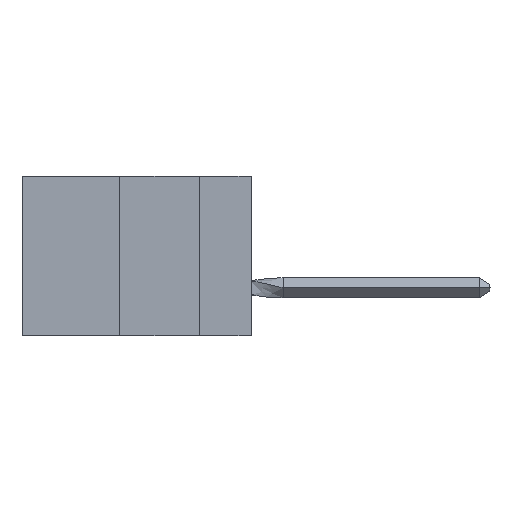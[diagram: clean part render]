
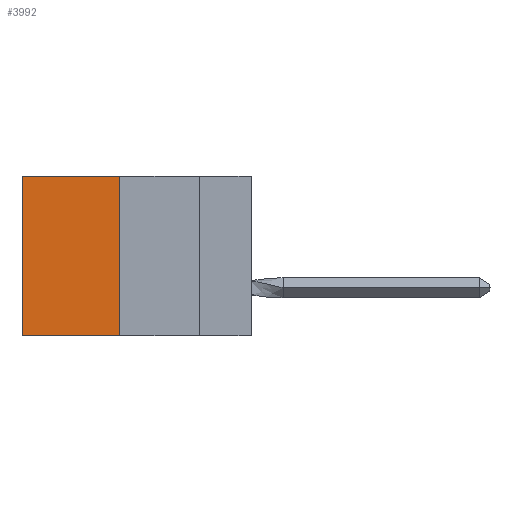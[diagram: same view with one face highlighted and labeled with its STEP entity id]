
A CAD part, left-side view. The second image highlights one B-rep face of the part: STEP entity #3992.
In plain terms, the highlighted planar face has unit normal (-1, 0, 0).
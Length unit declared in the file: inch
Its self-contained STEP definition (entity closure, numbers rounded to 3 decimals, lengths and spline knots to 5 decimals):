
#480 = VERTEX_POINT ( 'NONE', #12824 ) ;
#932 = PLANE ( 'NONE',  #18808 ) ;
#1014 = VERTEX_POINT ( 'NONE', #12391 ) ;
#2527 = ORIENTED_EDGE ( 'NONE', *, *, #12976, .T. ) ;
#2913 = DIRECTION ( 'NONE',  ( 0., 1., 0. ) ) ;
#2968 = CARTESIAN_POINT ( 'NONE',  ( 0.305, 0.413, -0.5 ) ) ;
#3451 = LINE ( 'NONE', #14095, #17153 ) ;
#3831 = DIRECTION ( 'NONE',  ( 0., 0., -1. ) ) ;
#3992 = ADVANCED_FACE ( 'NONE', ( #8481 ), #932, .F. ) ;
#5129 = CARTESIAN_POINT ( 'NONE',  ( 0.305, 0.413, -0.5 ) ) ;
#5790 = LINE ( 'NONE', #5129, #18299 ) ;
#6996 = ORIENTED_EDGE ( 'NONE', *, *, #18344, .F. ) ;
#7766 = DIRECTION ( 'NONE',  ( 0., 1., 0. ) ) ;
#8481 = FACE_OUTER_BOUND ( 'NONE', #9690, .T. ) ;
#9644 = VERTEX_POINT ( 'NONE', #10164 ) ;
#9690 = EDGE_LOOP ( 'NONE', ( #16705, #6996, #11796, #2527 ) ) ;
#10164 = CARTESIAN_POINT ( 'NONE',  ( 0.305, 0.72, 0. ) ) ;
#11166 = VECTOR ( 'NONE', #2913, 39.37008 ) ;
#11199 = CARTESIAN_POINT ( 'NONE',  ( 0.305, 0.413, -0.5 ) ) ;
#11796 = ORIENTED_EDGE ( 'NONE', *, *, #12617, .F. ) ;
#12078 = LINE ( 'NONE', #2968, #11166 ) ;
#12391 = CARTESIAN_POINT ( 'NONE',  ( 0.305, 0.413, -0.5 ) ) ;
#12617 = EDGE_CURVE ( 'NONE', #15176, #1014, #5790, .T. ) ;
#12824 = CARTESIAN_POINT ( 'NONE',  ( 0.305, 0.72, -0.5 ) ) ;
#12976 = EDGE_CURVE ( 'NONE', #15176, #9644, #14661, .T. ) ;
#13707 = CARTESIAN_POINT ( 'NONE',  ( 0.305, 0.413, 0. ) ) ;
#14095 = CARTESIAN_POINT ( 'NONE',  ( 0.305, 0.72, -0.5 ) ) ;
#14188 = DIRECTION ( 'NONE',  ( 1., 0., 0. ) ) ;
#14661 = LINE ( 'NONE', #13707, #16022 ) ;
#15176 = VERTEX_POINT ( 'NONE', #15998 ) ;
#15790 = DIRECTION ( 'NONE',  ( 0., 0., -1. ) ) ;
#15998 = CARTESIAN_POINT ( 'NONE',  ( 0.305, 0.413, 0. ) ) ;
#16022 = VECTOR ( 'NONE', #7766, 39.37008 ) ;
#16385 = EDGE_CURVE ( 'NONE', #9644, #480, #3451, .T. ) ;
#16705 = ORIENTED_EDGE ( 'NONE', *, *, #16385, .T. ) ;
#17000 = DIRECTION ( 'NONE',  ( 0., 0., -1. ) ) ;
#17153 = VECTOR ( 'NONE', #15790, 39.37008 ) ;
#18299 = VECTOR ( 'NONE', #17000, 39.37008 ) ;
#18344 = EDGE_CURVE ( 'NONE', #1014, #480, #12078, .T. ) ;
#18808 = AXIS2_PLACEMENT_3D ( 'NONE', #11199, #14188, #3831 ) ;
